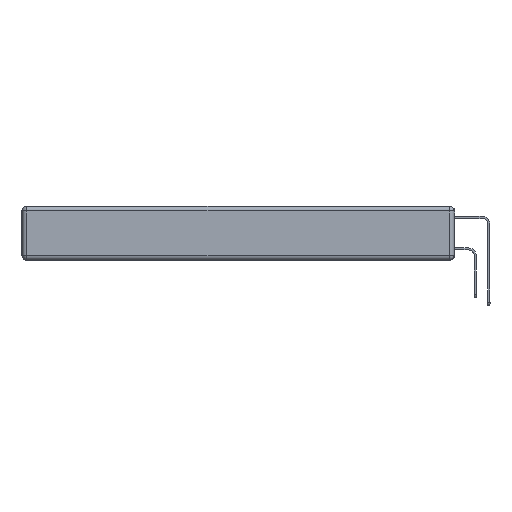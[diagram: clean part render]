
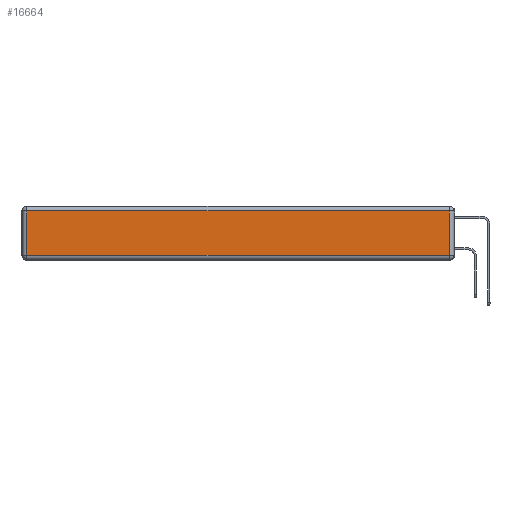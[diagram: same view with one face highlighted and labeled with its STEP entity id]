
A CAD part, left-side view. The second image highlights one B-rep face of the part: STEP entity #16664.
In plain terms, the highlighted planar face has unit normal (-1, 0, 0).
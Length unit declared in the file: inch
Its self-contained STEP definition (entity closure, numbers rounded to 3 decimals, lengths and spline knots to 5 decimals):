
#257 = CARTESIAN_POINT ( 'NONE',  ( 0., 2.75, -0.03 ) ) ;
#824 = EDGE_LOOP ( 'NONE', ( #8682, #20738, #9043, #4796 ) ) ;
#1424 = CARTESIAN_POINT ( 'NONE',  ( 0., 0.03, -0.03 ) ) ;
#2130 = DIRECTION ( 'NONE',  ( 0., 1., 0. ) ) ;
#2384 = LINE ( 'NONE', #21239, #15471 ) ;
#2729 = CARTESIAN_POINT ( 'NONE',  ( 0., 0., -0.313 ) ) ;
#3019 = CARTESIAN_POINT ( 'NONE',  ( 0., 0., -0.343 ) ) ;
#4245 = EDGE_CURVE ( 'NONE', #17573, #10380, #10557, .T. ) ;
#4366 = VERTEX_POINT ( 'NONE', #8474 ) ;
#4483 = CARTESIAN_POINT ( 'NONE',  ( 0., 2.72, -0.343 ) ) ;
#4796 = ORIENTED_EDGE ( 'NONE', *, *, #19795, .T. ) ;
#6207 = DIRECTION ( 'NONE',  ( 0., 0., 1. ) ) ;
#7544 = DIRECTION ( 'NONE',  ( 0., -1., 0. ) ) ;
#8192 = EDGE_CURVE ( 'NONE', #20157, #17573, #2384, .T. ) ;
#8474 = CARTESIAN_POINT ( 'NONE',  ( 0., 2.72, -0.313 ) ) ;
#8682 = ORIENTED_EDGE ( 'NONE', *, *, #14509, .T. ) ;
#9043 = ORIENTED_EDGE ( 'NONE', *, *, #4245, .T. ) ;
#9357 = VECTOR ( 'NONE', #2130, 39.37008 ) ;
#9956 = CARTESIAN_POINT ( 'NONE',  ( 0., 2.72, -0.03 ) ) ;
#10115 = PLANE ( 'NONE',  #10832 ) ;
#10380 = VERTEX_POINT ( 'NONE', #9956 ) ;
#10483 = CARTESIAN_POINT ( 'NONE',  ( 0., 0.03, -0.313 ) ) ;
#10557 = LINE ( 'NONE', #257, #9357 ) ;
#10832 = AXIS2_PLACEMENT_3D ( 'NONE', #3019, #18433, #21531 ) ;
#12916 = DIRECTION ( 'NONE',  ( 0., 0., -1. ) ) ;
#13414 = FACE_OUTER_BOUND ( 'NONE', #824, .T. ) ;
#13904 = VECTOR ( 'NONE', #7544, 39.37008 ) ;
#14509 = EDGE_CURVE ( 'NONE', #4366, #20157, #19590, .T. ) ;
#14705 = VECTOR ( 'NONE', #12916, 39.37008 ) ;
#15471 = VECTOR ( 'NONE', #6207, 39.37008 ) ;
#16664 = ADVANCED_FACE ( 'NONE', ( #13414 ), #10115, .T. ) ;
#17573 = VERTEX_POINT ( 'NONE', #1424 ) ;
#18433 = DIRECTION ( 'NONE',  ( -1., 0., 0. ) ) ;
#19486 = LINE ( 'NONE', #4483, #14705 ) ;
#19590 = LINE ( 'NONE', #2729, #13904 ) ;
#19795 = EDGE_CURVE ( 'NONE', #10380, #4366, #19486, .T. ) ;
#20157 = VERTEX_POINT ( 'NONE', #10483 ) ;
#20738 = ORIENTED_EDGE ( 'NONE', *, *, #8192, .T. ) ;
#21239 = CARTESIAN_POINT ( 'NONE',  ( 0., 0.03, -0.343 ) ) ;
#21531 = DIRECTION ( 'NONE',  ( 0., 0., 1. ) ) ;
